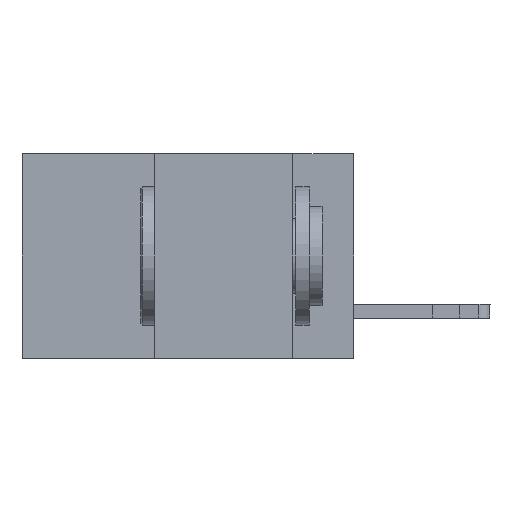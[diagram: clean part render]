
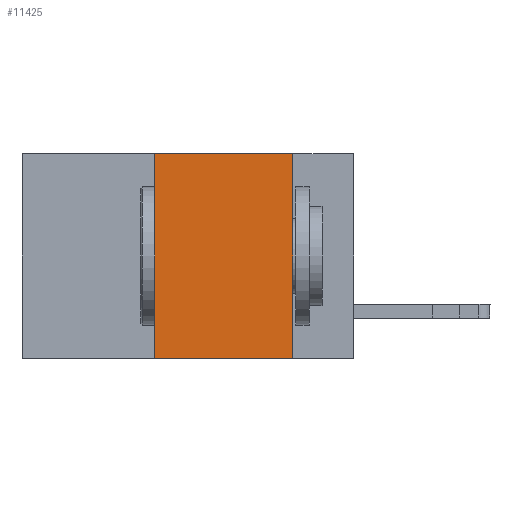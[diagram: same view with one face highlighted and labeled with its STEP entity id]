
A CAD part, left-side view. The second image highlights one B-rep face of the part: STEP entity #11425.
In plain terms, the highlighted planar face has unit normal (-1, 0, 0).
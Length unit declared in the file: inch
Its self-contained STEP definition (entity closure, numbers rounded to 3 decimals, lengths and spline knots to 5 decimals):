
#646 = LINE ( 'NONE', #5245, #14785 ) ;
#673 = VERTEX_POINT ( 'NONE', #13077 ) ;
#1011 = CARTESIAN_POINT ( 'NONE',  ( 0., 0.11, -0.37 ) ) ;
#1407 = ORIENTED_EDGE ( 'NONE', *, *, #13302, .F. ) ;
#1473 = LINE ( 'NONE', #3119, #13656 ) ;
#1652 = PLANE ( 'NONE',  #14896 ) ;
#2785 = DIRECTION ( 'NONE',  ( 0., 0., -1. ) ) ;
#3119 = CARTESIAN_POINT ( 'NONE',  ( 0., 0.6, 0. ) ) ;
#3963 = CARTESIAN_POINT ( 'NONE',  ( 0., 0.11, 0. ) ) ;
#4153 = VERTEX_POINT ( 'NONE', #1011 ) ;
#4520 = LINE ( 'NONE', #3963, #10826 ) ;
#5245 = CARTESIAN_POINT ( 'NONE',  ( 0., 0.36, 0. ) ) ;
#6005 = ORIENTED_EDGE ( 'NONE', *, *, #14705, .F. ) ;
#6757 = ORIENTED_EDGE ( 'NONE', *, *, #7702, .T. ) ;
#6777 = DIRECTION ( 'NONE',  ( 0., 0., 1. ) ) ;
#7077 = DIRECTION ( 'NONE',  ( 0., -1., 0. ) ) ;
#7702 = EDGE_CURVE ( 'NONE', #673, #4153, #11760, .T. ) ;
#7794 = EDGE_LOOP ( 'NONE', ( #1407, #14566, #6005, #6757 ) ) ;
#7857 = CARTESIAN_POINT ( 'NONE',  ( 0., 0.6, 0. ) ) ;
#8887 = CARTESIAN_POINT ( 'NONE',  ( 0., 0.36, 0. ) ) ;
#10806 = VERTEX_POINT ( 'NONE', #8887 ) ;
#10826 = VECTOR ( 'NONE', #12764, 39.37008 ) ;
#11425 = ADVANCED_FACE ( 'NONE', ( #12054 ), #1652, .F. ) ;
#11760 = LINE ( 'NONE', #12950, #15681 ) ;
#11946 = EDGE_CURVE ( 'NONE', #10806, #16126, #1473, .T. ) ;
#12054 = FACE_OUTER_BOUND ( 'NONE', #7794, .T. ) ;
#12764 = DIRECTION ( 'NONE',  ( 0., 0., -1. ) ) ;
#12895 = DIRECTION ( 'NONE',  ( 1., 0., 0. ) ) ;
#12950 = CARTESIAN_POINT ( 'NONE',  ( 0., 0.6, -0.37 ) ) ;
#13077 = CARTESIAN_POINT ( 'NONE',  ( 0., 0.36, -0.37 ) ) ;
#13302 = EDGE_CURVE ( 'NONE', #16126, #4153, #4520, .T. ) ;
#13656 = VECTOR ( 'NONE', #7077, 39.37008 ) ;
#14081 = DIRECTION ( 'NONE',  ( 0., -1., 0. ) ) ;
#14119 = CARTESIAN_POINT ( 'NONE',  ( 0., 0.11, 0. ) ) ;
#14566 = ORIENTED_EDGE ( 'NONE', *, *, #11946, .F. ) ;
#14705 = EDGE_CURVE ( 'NONE', #673, #10806, #646, .T. ) ;
#14785 = VECTOR ( 'NONE', #6777, 39.37008 ) ;
#14896 = AXIS2_PLACEMENT_3D ( 'NONE', #7857, #12895, #2785 ) ;
#15681 = VECTOR ( 'NONE', #14081, 39.37008 ) ;
#16126 = VERTEX_POINT ( 'NONE', #14119 ) ;
